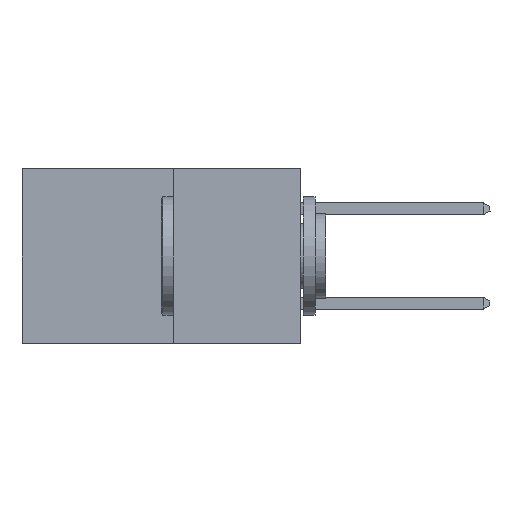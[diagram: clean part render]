
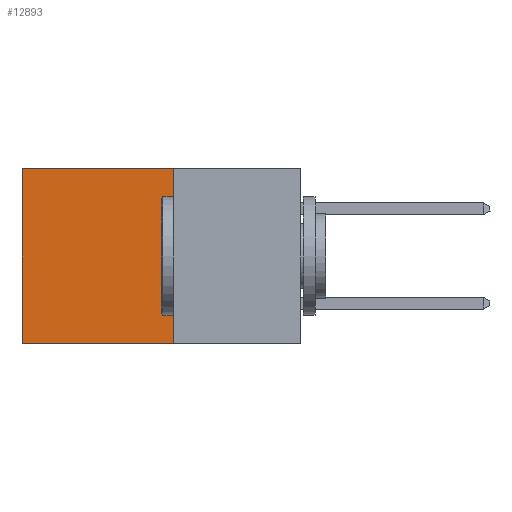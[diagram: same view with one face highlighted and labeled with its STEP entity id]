
A CAD part, left-side view. The second image highlights one B-rep face of the part: STEP entity #12893.
In plain terms, the highlighted planar face has unit normal (-1, 0, 0).
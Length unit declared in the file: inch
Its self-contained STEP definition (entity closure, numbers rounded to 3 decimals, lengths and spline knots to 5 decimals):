
#947 = DIRECTION ( 'NONE',  ( 0., 1., 0. ) ) ;
#1563 = VECTOR ( 'NONE', #947, 39.37008 ) ;
#1577 = EDGE_CURVE ( 'NONE', #17230, #18354, #10641, .T. ) ;
#3389 = CARTESIAN_POINT ( 'NONE',  ( 0.277, 0.59, 0. ) ) ;
#3740 = CARTESIAN_POINT ( 'NONE',  ( 0.277, 0.27, 0. ) ) ;
#3879 = EDGE_CURVE ( 'NONE', #27209, #6150, #25342, .T. ) ;
#5195 = CARTESIAN_POINT ( 'NONE',  ( 0.277, 0.27, -0.37 ) ) ;
#5710 = CARTESIAN_POINT ( 'NONE',  ( 0.277, 0.27, -0.37 ) ) ;
#6150 = VERTEX_POINT ( 'NONE', #9791 ) ;
#6471 = ORIENTED_EDGE ( 'NONE', *, *, #17605, .F. ) ;
#6504 = LINE ( 'NONE', #5195, #1563 ) ;
#6764 = DIRECTION ( 'NONE',  ( 0., 0., -1. ) ) ;
#6966 = CARTESIAN_POINT ( 'NONE',  ( 0.277, 0.59, -0.37 ) ) ;
#8415 = CARTESIAN_POINT ( 'NONE',  ( 0.277, 0.27, 0. ) ) ;
#9132 = VECTOR ( 'NONE', #12938, 39.37008 ) ;
#9791 = CARTESIAN_POINT ( 'NONE',  ( 0.277, 0.59, -0.37 ) ) ;
#10641 = LINE ( 'NONE', #13712, #9132 ) ;
#11864 = ORIENTED_EDGE ( 'NONE', *, *, #3879, .T. ) ;
#11908 = CARTESIAN_POINT ( 'NONE',  ( 0.277, 0.27, -0.37 ) ) ;
#12262 = ORIENTED_EDGE ( 'NONE', *, *, #15702, .T. ) ;
#12893 = ADVANCED_FACE ( 'NONE', ( #23526 ), #24961, .F. ) ;
#12938 = DIRECTION ( 'NONE',  ( 0., 0., -1. ) ) ;
#13292 = AXIS2_PLACEMENT_3D ( 'NONE', #5710, #27088, #14336 ) ;
#13712 = CARTESIAN_POINT ( 'NONE',  ( 0.277, 0.27, -0.37 ) ) ;
#14336 = DIRECTION ( 'NONE',  ( 0., 0., -1. ) ) ;
#15702 = EDGE_CURVE ( 'NONE', #17230, #27209, #23993, .T. ) ;
#17230 = VERTEX_POINT ( 'NONE', #8415 ) ;
#17248 = ORIENTED_EDGE ( 'NONE', *, *, #1577, .F. ) ;
#17605 = EDGE_CURVE ( 'NONE', #18354, #6150, #6504, .T. ) ;
#18354 = VERTEX_POINT ( 'NONE', #11908 ) ;
#18972 = VECTOR ( 'NONE', #20829, 39.37008 ) ;
#19219 = EDGE_LOOP ( 'NONE', ( #11864, #6471, #17248, #12262 ) ) ;
#20829 = DIRECTION ( 'NONE',  ( 0., 1., 0. ) ) ;
#23352 = VECTOR ( 'NONE', #6764, 39.37008 ) ;
#23526 = FACE_OUTER_BOUND ( 'NONE', #19219, .T. ) ;
#23993 = LINE ( 'NONE', #3740, #18972 ) ;
#24961 = PLANE ( 'NONE',  #13292 ) ;
#25342 = LINE ( 'NONE', #6966, #23352 ) ;
#27088 = DIRECTION ( 'NONE',  ( 1., 0., 0. ) ) ;
#27209 = VERTEX_POINT ( 'NONE', #3389 ) ;
